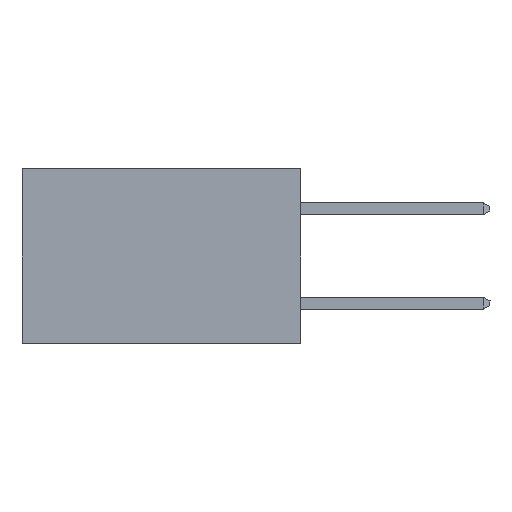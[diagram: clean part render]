
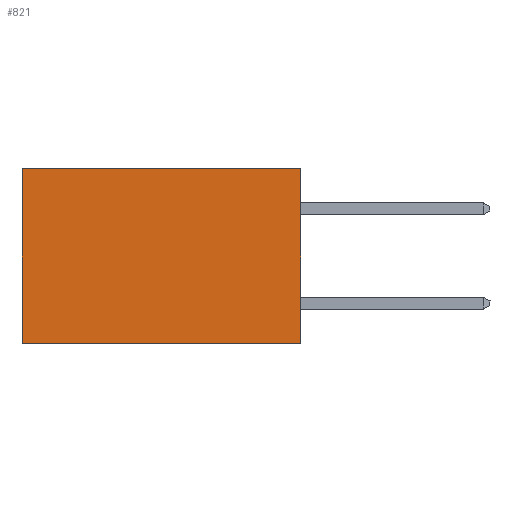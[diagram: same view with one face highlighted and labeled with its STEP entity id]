
A CAD part, left-side view. The second image highlights one B-rep face of the part: STEP entity #821.
In plain terms, the highlighted planar face has unit normal (-1, 0, 0).
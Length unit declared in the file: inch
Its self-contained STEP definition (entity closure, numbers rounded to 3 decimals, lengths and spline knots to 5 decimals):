
#821 = ADVANCED_FACE ( 'NONE', ( #27258 ), #12781, .F. ) ;
#1097 = LINE ( 'NONE', #17952, #23002 ) ;
#1192 = EDGE_CURVE ( 'NONE', #21163, #22595, #1649, .T. ) ;
#1649 = LINE ( 'NONE', #16937, #24232 ) ;
#5088 = EDGE_CURVE ( 'NONE', #21163, #10220, #1097, .T. ) ;
#5858 = CARTESIAN_POINT ( 'NONE',  ( 0.277, 0., -0.37 ) ) ;
#5946 = DIRECTION ( 'NONE',  ( 0., 0., -1. ) ) ;
#6318 = ORIENTED_EDGE ( 'NONE', *, *, #1192, .T. ) ;
#6467 = LINE ( 'NONE', #25110, #23835 ) ;
#7696 = LINE ( 'NONE', #22043, #24377 ) ;
#8997 = CARTESIAN_POINT ( 'NONE',  ( 0.277, 0.59, -0.37 ) ) ;
#9890 = DIRECTION ( 'NONE',  ( 0., 0., -1. ) ) ;
#9982 = DIRECTION ( 'NONE',  ( 0., 1., 0. ) ) ;
#10220 = VERTEX_POINT ( 'NONE', #5858 ) ;
#11230 = ORIENTED_EDGE ( 'NONE', *, *, #17212, .T. ) ;
#11637 = DIRECTION ( 'NONE',  ( 1., 0., 0. ) ) ;
#11835 = CARTESIAN_POINT ( 'NONE',  ( 0.277, 0., -0.37 ) ) ;
#12781 = PLANE ( 'NONE',  #16132 ) ;
#15525 = DIRECTION ( 'NONE',  ( 0., 1., 0. ) ) ;
#16132 = AXIS2_PLACEMENT_3D ( 'NONE', #11835, #11637, #5946 ) ;
#16937 = CARTESIAN_POINT ( 'NONE',  ( 0.277, 0., 0. ) ) ;
#17067 = ORIENTED_EDGE ( 'NONE', *, *, #20651, .F. ) ;
#17212 = EDGE_CURVE ( 'NONE', #22595, #25766, #6467, .T. ) ;
#17709 = DIRECTION ( 'NONE',  ( 0., 0., -1. ) ) ;
#17952 = CARTESIAN_POINT ( 'NONE',  ( 0.277, 0., -0.37 ) ) ;
#19061 = CARTESIAN_POINT ( 'NONE',  ( 0.277, 0., 0. ) ) ;
#20651 = EDGE_CURVE ( 'NONE', #10220, #25766, #7696, .T. ) ;
#21163 = VERTEX_POINT ( 'NONE', #19061 ) ;
#21773 = ORIENTED_EDGE ( 'NONE', *, *, #5088, .F. ) ;
#22043 = CARTESIAN_POINT ( 'NONE',  ( 0.277, 0., -0.37 ) ) ;
#22595 = VERTEX_POINT ( 'NONE', #23825 ) ;
#23002 = VECTOR ( 'NONE', #17709, 39.37008 ) ;
#23825 = CARTESIAN_POINT ( 'NONE',  ( 0.277, 0.59, 0. ) ) ;
#23835 = VECTOR ( 'NONE', #9890, 39.37008 ) ;
#24232 = VECTOR ( 'NONE', #9982, 39.37008 ) ;
#24377 = VECTOR ( 'NONE', #15525, 39.37008 ) ;
#25110 = CARTESIAN_POINT ( 'NONE',  ( 0.277, 0.59, -0.37 ) ) ;
#25766 = VERTEX_POINT ( 'NONE', #8997 ) ;
#27258 = FACE_OUTER_BOUND ( 'NONE', #28150, .T. ) ;
#28150 = EDGE_LOOP ( 'NONE', ( #11230, #17067, #21773, #6318 ) ) ;
